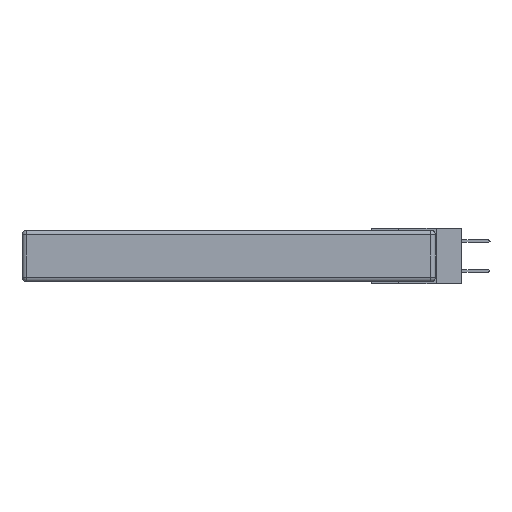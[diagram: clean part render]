
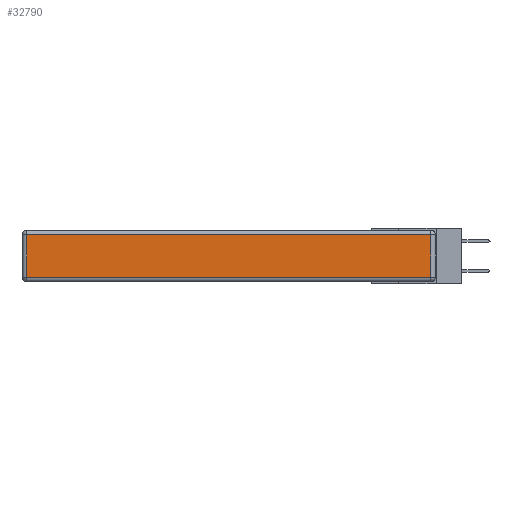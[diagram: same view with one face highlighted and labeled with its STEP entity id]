
A CAD part, left-side view. The second image highlights one B-rep face of the part: STEP entity #32790.
In plain terms, the highlighted planar face has unit normal (-1, 0, 0).
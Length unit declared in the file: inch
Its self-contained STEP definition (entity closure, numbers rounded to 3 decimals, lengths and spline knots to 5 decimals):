
#1188 = VERTEX_POINT ( 'NONE', #11187 ) ;
#3020 = LINE ( 'NONE', #15068, #20912 ) ;
#3777 = CARTESIAN_POINT ( 'NONE',  ( 0., 2.75, -0.03 ) ) ;
#4691 = EDGE_CURVE ( 'NONE', #11507, #17299, #3020, .T. ) ;
#10647 = VECTOR ( 'NONE', #14368, 39.37008 ) ;
#10913 = CARTESIAN_POINT ( 'NONE',  ( 0., 2.72, -0.343 ) ) ;
#11186 = ORIENTED_EDGE ( 'NONE', *, *, #31311, .T. ) ;
#11187 = CARTESIAN_POINT ( 'NONE',  ( 0., 0.03, -0.03 ) ) ;
#11507 = VERTEX_POINT ( 'NONE', #19652 ) ;
#11865 = AXIS2_PLACEMENT_3D ( 'NONE', #27340, #27461, #17146 ) ;
#14368 = DIRECTION ( 'NONE',  ( 0., 0., -1. ) ) ;
#14539 = PLANE ( 'NONE',  #11865 ) ;
#14786 = LINE ( 'NONE', #18343, #33052 ) ;
#15068 = CARTESIAN_POINT ( 'NONE',  ( 0., 0., -0.313 ) ) ;
#16447 = VECTOR ( 'NONE', #16752, 39.37008 ) ;
#16752 = DIRECTION ( 'NONE',  ( 0., 1., 0. ) ) ;
#17146 = DIRECTION ( 'NONE',  ( 0., 0., 1. ) ) ;
#17299 = VERTEX_POINT ( 'NONE', #17911 ) ;
#17316 = EDGE_CURVE ( 'NONE', #17299, #1188, #14786, .T. ) ;
#17911 = CARTESIAN_POINT ( 'NONE',  ( 0., 0.03, -0.313 ) ) ;
#18343 = CARTESIAN_POINT ( 'NONE',  ( 0., 0.03, -0.343 ) ) ;
#19652 = CARTESIAN_POINT ( 'NONE',  ( 0., 2.72, -0.313 ) ) ;
#20270 = DIRECTION ( 'NONE',  ( 0., -1., 0. ) ) ;
#20530 = ORIENTED_EDGE ( 'NONE', *, *, #4691, .T. ) ;
#20912 = VECTOR ( 'NONE', #20270, 39.37008 ) ;
#23372 = DIRECTION ( 'NONE',  ( 0., 0., 1. ) ) ;
#23648 = VERTEX_POINT ( 'NONE', #28539 ) ;
#24045 = FACE_OUTER_BOUND ( 'NONE', #32116, .T. ) ;
#24429 = LINE ( 'NONE', #10913, #10647 ) ;
#24926 = ORIENTED_EDGE ( 'NONE', *, *, #17316, .T. ) ;
#25287 = EDGE_CURVE ( 'NONE', #23648, #11507, #24429, .T. ) ;
#25392 = ORIENTED_EDGE ( 'NONE', *, *, #25287, .T. ) ;
#27340 = CARTESIAN_POINT ( 'NONE',  ( 0., 0., -0.343 ) ) ;
#27461 = DIRECTION ( 'NONE',  ( -1., 0., 0. ) ) ;
#28539 = CARTESIAN_POINT ( 'NONE',  ( 0., 2.72, -0.03 ) ) ;
#31311 = EDGE_CURVE ( 'NONE', #1188, #23648, #31462, .T. ) ;
#31462 = LINE ( 'NONE', #3777, #16447 ) ;
#32116 = EDGE_LOOP ( 'NONE', ( #20530, #24926, #11186, #25392 ) ) ;
#32790 = ADVANCED_FACE ( 'NONE', ( #24045 ), #14539, .T. ) ;
#33052 = VECTOR ( 'NONE', #23372, 39.37008 ) ;
